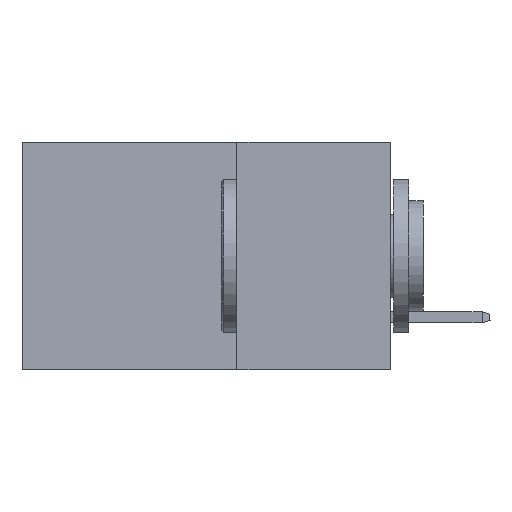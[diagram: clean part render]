
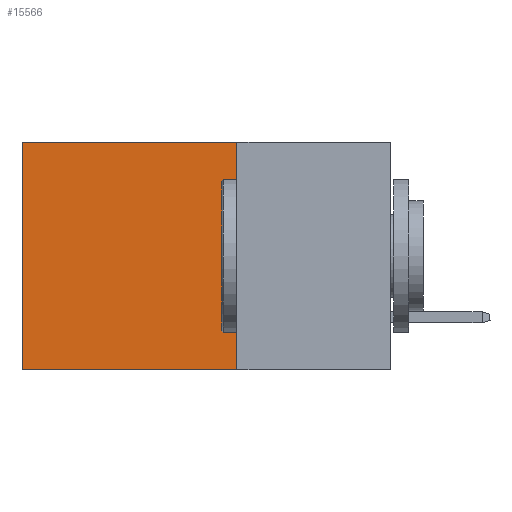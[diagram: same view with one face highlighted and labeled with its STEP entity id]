
A CAD part, left-side view. The second image highlights one B-rep face of the part: STEP entity #15566.
In plain terms, the highlighted planar face has unit normal (-1, 0, 0).
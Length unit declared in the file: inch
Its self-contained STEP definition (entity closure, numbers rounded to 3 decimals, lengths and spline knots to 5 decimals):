
#980 = CARTESIAN_POINT ( 'NONE',  ( 0.2875, 0.25, -0.37 ) ) ;
#1318 = FACE_OUTER_BOUND ( 'NONE', #28451, .T. ) ;
#2702 = EDGE_CURVE ( 'NONE', #6867, #11835, #20202, .T. ) ;
#3522 = VERTEX_POINT ( 'NONE', #15340 ) ;
#3863 = LINE ( 'NONE', #7779, #32226 ) ;
#4587 = ORIENTED_EDGE ( 'NONE', *, *, #36799, .F. ) ;
#4639 = VECTOR ( 'NONE', #30507, 39.37008 ) ;
#6867 = VERTEX_POINT ( 'NONE', #26689 ) ;
#7020 = DIRECTION ( 'NONE',  ( 0., 1., 0. ) ) ;
#7150 = DIRECTION ( 'NONE',  ( 0., 0., -1. ) ) ;
#7292 = VECTOR ( 'NONE', #7020, 39.37008 ) ;
#7779 = CARTESIAN_POINT ( 'NONE',  ( 0.2875, 0.6, 0. ) ) ;
#7873 = AXIS2_PLACEMENT_3D ( 'NONE', #18790, #24640, #7150 ) ;
#8571 = ORIENTED_EDGE ( 'NONE', *, *, #15560, .T. ) ;
#10073 = PLANE ( 'NONE',  #7873 ) ;
#11835 = VERTEX_POINT ( 'NONE', #980 ) ;
#13361 = DIRECTION ( 'NONE',  ( 0., 0., -1. ) ) ;
#13839 = CARTESIAN_POINT ( 'NONE',  ( 0.2875, 0.25, -0.37 ) ) ;
#14632 = ORIENTED_EDGE ( 'NONE', *, *, #27963, .T. ) ;
#14820 = VECTOR ( 'NONE', #37120, 39.37008 ) ;
#15340 = CARTESIAN_POINT ( 'NONE',  ( 0.2875, 0.6, 0. ) ) ;
#15560 = EDGE_CURVE ( 'NONE', #6867, #3522, #27874, .T. ) ;
#15566 = ADVANCED_FACE ( 'NONE', ( #1318 ), #10073, .F. ) ;
#18384 = CARTESIAN_POINT ( 'NONE',  ( 0.2875, 0.25, 0. ) ) ;
#18790 = CARTESIAN_POINT ( 'NONE',  ( 0.2875, 0.25, 0. ) ) ;
#20202 = LINE ( 'NONE', #18384, #4639 ) ;
#20737 = CARTESIAN_POINT ( 'NONE',  ( 0.2875, 0.6, -0.37 ) ) ;
#24515 = CARTESIAN_POINT ( 'NONE',  ( 0.2875, 0.25, 0. ) ) ;
#24640 = DIRECTION ( 'NONE',  ( 1., 0., 0. ) ) ;
#26689 = CARTESIAN_POINT ( 'NONE',  ( 0.2875, 0.25, 0. ) ) ;
#27073 = VERTEX_POINT ( 'NONE', #20737 ) ;
#27483 = ORIENTED_EDGE ( 'NONE', *, *, #2702, .F. ) ;
#27874 = LINE ( 'NONE', #24515, #7292 ) ;
#27963 = EDGE_CURVE ( 'NONE', #3522, #27073, #3863, .T. ) ;
#28451 = EDGE_LOOP ( 'NONE', ( #14632, #4587, #27483, #8571 ) ) ;
#30507 = DIRECTION ( 'NONE',  ( 0., 0., -1. ) ) ;
#32226 = VECTOR ( 'NONE', #13361, 39.37008 ) ;
#32234 = LINE ( 'NONE', #13839, #14820 ) ;
#36799 = EDGE_CURVE ( 'NONE', #11835, #27073, #32234, .T. ) ;
#37120 = DIRECTION ( 'NONE',  ( 0., 1., 0. ) ) ;
